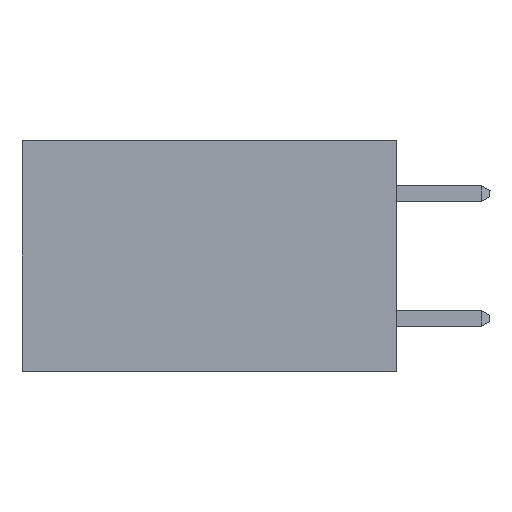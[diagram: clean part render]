
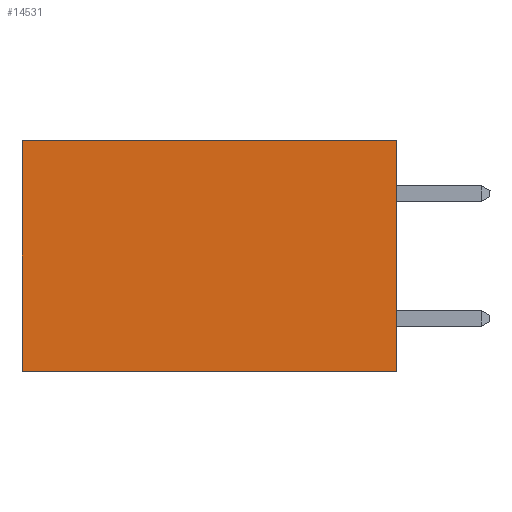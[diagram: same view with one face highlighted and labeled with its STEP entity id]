
A CAD part, left-side view. The second image highlights one B-rep face of the part: STEP entity #14531.
In plain terms, the highlighted planar face has unit normal (-1, 0, 0).
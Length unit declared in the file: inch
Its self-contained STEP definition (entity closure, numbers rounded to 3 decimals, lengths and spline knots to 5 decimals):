
#560 = AXIS2_PLACEMENT_3D ( 'NONE', #23516, #25726, #16151 ) ;
#1758 = PLANE ( 'NONE',  #560 ) ;
#2099 = VECTOR ( 'NONE', #25868, 39.37008 ) ;
#2153 = ORIENTED_EDGE ( 'NONE', *, *, #19020, .F. ) ;
#4789 = ORIENTED_EDGE ( 'NONE', *, *, #21492, .T. ) ;
#6309 = CARTESIAN_POINT ( 'NONE',  ( 0.298, 0.6, -0.37 ) ) ;
#7566 = VECTOR ( 'NONE', #13771, 39.37008 ) ;
#8313 = LINE ( 'NONE', #28157, #7566 ) ;
#9089 = CARTESIAN_POINT ( 'NONE',  ( 0.298, 0.6, 0. ) ) ;
#9560 = VECTOR ( 'NONE', #14106, 39.37008 ) ;
#10157 = VERTEX_POINT ( 'NONE', #18456 ) ;
#10513 = FACE_OUTER_BOUND ( 'NONE', #13830, .T. ) ;
#10578 = CARTESIAN_POINT ( 'NONE',  ( 0.298, 0., 0. ) ) ;
#11575 = EDGE_CURVE ( 'NONE', #16079, #17393, #20454, .T. ) ;
#13771 = DIRECTION ( 'NONE',  ( 0., 0., -1. ) ) ;
#13830 = EDGE_LOOP ( 'NONE', ( #30515, #24870, #2153, #4789 ) ) ;
#14106 = DIRECTION ( 'NONE',  ( 0., 1., 0. ) ) ;
#14531 = ADVANCED_FACE ( 'NONE', ( #10513 ), #1758, .F. ) ;
#15961 = DIRECTION ( 'NONE',  ( 0., 1., 0. ) ) ;
#16079 = VERTEX_POINT ( 'NONE', #16723 ) ;
#16151 = DIRECTION ( 'NONE',  ( 0., 0., -1. ) ) ;
#16464 = EDGE_CURVE ( 'NONE', #10157, #17393, #28358, .T. ) ;
#16723 = CARTESIAN_POINT ( 'NONE',  ( 0.298, 0.6, 0. ) ) ;
#17393 = VERTEX_POINT ( 'NONE', #6309 ) ;
#18213 = VECTOR ( 'NONE', #15961, 39.37008 ) ;
#18456 = CARTESIAN_POINT ( 'NONE',  ( 0.298, 0., -0.37 ) ) ;
#19020 = EDGE_CURVE ( 'NONE', #26928, #10157, #8313, .T. ) ;
#20454 = LINE ( 'NONE', #9089, #2099 ) ;
#20786 = LINE ( 'NONE', #21257, #9560 ) ;
#21257 = CARTESIAN_POINT ( 'NONE',  ( 0.298, 0., 0. ) ) ;
#21492 = EDGE_CURVE ( 'NONE', #26928, #16079, #20786, .T. ) ;
#23516 = CARTESIAN_POINT ( 'NONE',  ( 0.298, 0., 0. ) ) ;
#24870 = ORIENTED_EDGE ( 'NONE', *, *, #16464, .F. ) ;
#25726 = DIRECTION ( 'NONE',  ( 1., 0., 0. ) ) ;
#25868 = DIRECTION ( 'NONE',  ( 0., 0., -1. ) ) ;
#26928 = VERTEX_POINT ( 'NONE', #10578 ) ;
#28157 = CARTESIAN_POINT ( 'NONE',  ( 0.298, 0., 0. ) ) ;
#28358 = LINE ( 'NONE', #30381, #18213 ) ;
#30381 = CARTESIAN_POINT ( 'NONE',  ( 0.298, 0., -0.37 ) ) ;
#30515 = ORIENTED_EDGE ( 'NONE', *, *, #11575, .T. ) ;
